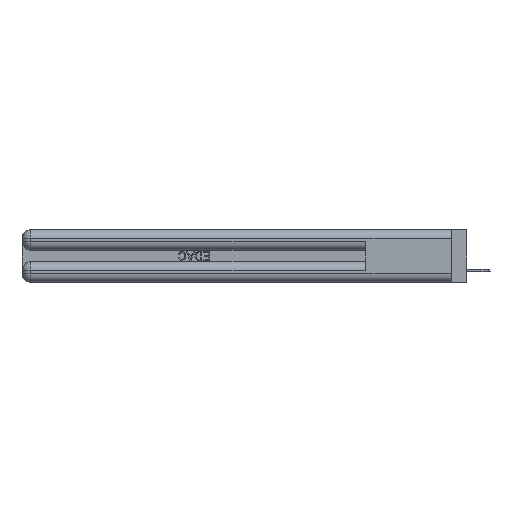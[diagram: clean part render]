
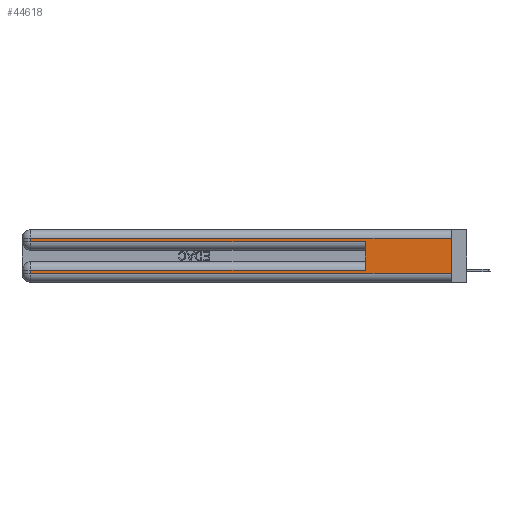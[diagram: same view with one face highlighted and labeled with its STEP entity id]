
A CAD part, left-side view. The second image highlights one B-rep face of the part: STEP entity #44618.
In plain terms, the highlighted planar face has unit normal (-1, 0, 0).
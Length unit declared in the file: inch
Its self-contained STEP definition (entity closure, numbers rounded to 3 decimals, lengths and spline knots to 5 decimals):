
#7 = EDGE_CURVE ( 'NONE', #6114, #13616, #32030, .T. ) ;
#2860 = DIRECTION ( 'NONE',  ( 0., 0., -1. ) ) ;
#5725 = VERTEX_POINT ( 'NONE', #36830 ) ;
#6114 = VERTEX_POINT ( 'NONE', #42309 ) ;
#8122 = EDGE_LOOP ( 'NONE', ( #51511, #28644, #48991, #49494, #27623, #25606, #29143, #9548 ) ) ;
#8180 = LINE ( 'NONE', #36721, #25839 ) ;
#8453 = VECTOR ( 'NONE', #35590, 39.37008 ) ;
#9548 = ORIENTED_EDGE ( 'NONE', *, *, #47513, .T. ) ;
#10100 = CARTESIAN_POINT ( 'NONE',  ( 0., 2.94, 0.37 ) ) ;
#11999 = EDGE_CURVE ( 'NONE', #47653, #46898, #13124, .T. ) ;
#12465 = VECTOR ( 'NONE', #18712, 39.37008 ) ;
#13124 = LINE ( 'NONE', #14796, #12465 ) ;
#13616 = VERTEX_POINT ( 'NONE', #33206 ) ;
#14796 = CARTESIAN_POINT ( 'NONE',  ( 0., 0., 0.285 ) ) ;
#15668 = VECTOR ( 'NONE', #39580, 39.37008 ) ;
#16251 = FACE_OUTER_BOUND ( 'NONE', #8122, .T. ) ;
#17069 = VECTOR ( 'NONE', #31730, 39.37008 ) ;
#17251 = CARTESIAN_POINT ( 'NONE',  ( 0., 2.94, 0.285 ) ) ;
#17405 = EDGE_CURVE ( 'NONE', #5725, #22506, #32614, .T. ) ;
#18120 = VERTEX_POINT ( 'NONE', #48174 ) ;
#18712 = DIRECTION ( 'NONE',  ( 0., -1., 0. ) ) ;
#22506 = VERTEX_POINT ( 'NONE', #42039 ) ;
#23694 = LINE ( 'NONE', #38310, #8453 ) ;
#24820 = EDGE_CURVE ( 'NONE', #13616, #44386, #34417, .T. ) ;
#24908 = EDGE_CURVE ( 'NONE', #6114, #46898, #23694, .T. ) ;
#25606 = ORIENTED_EDGE ( 'NONE', *, *, #7, .T. ) ;
#25839 = VECTOR ( 'NONE', #28259, 39.37008 ) ;
#27623 = ORIENTED_EDGE ( 'NONE', *, *, #24908, .F. ) ;
#27750 = CARTESIAN_POINT ( 'NONE',  ( 0., 2.94, 0.37 ) ) ;
#28259 = DIRECTION ( 'NONE',  ( 0., 0., -1. ) ) ;
#28539 = EDGE_CURVE ( 'NONE', #22506, #47653, #52403, .T. ) ;
#28644 = ORIENTED_EDGE ( 'NONE', *, *, #17405, .T. ) ;
#29143 = ORIENTED_EDGE ( 'NONE', *, *, #24820, .T. ) ;
#31730 = DIRECTION ( 'NONE',  ( 0., -1., 0. ) ) ;
#32030 = LINE ( 'NONE', #43398, #47993 ) ;
#32614 = LINE ( 'NONE', #51875, #15668 ) ;
#33206 = CARTESIAN_POINT ( 'NONE',  ( 0., 2.94, 0.085 ) ) ;
#33969 = DIRECTION ( 'NONE',  ( 1., 0., 0. ) ) ;
#34417 = LINE ( 'NONE', #27750, #50307 ) ;
#34623 = AXIS2_PLACEMENT_3D ( 'NONE', #49252, #33969, #50313 ) ;
#35590 = DIRECTION ( 'NONE',  ( 0., 0., 1. ) ) ;
#36721 = CARTESIAN_POINT ( 'NONE',  ( 0., 0., 0.37 ) ) ;
#36725 = LINE ( 'NONE', #44686, #17069 ) ;
#36830 = CARTESIAN_POINT ( 'NONE',  ( 0., 0., 0.31 ) ) ;
#38310 = CARTESIAN_POINT ( 'NONE',  ( 0., 0.6, 0.145 ) ) ;
#39560 = CARTESIAN_POINT ( 'NONE',  ( 0., 2.94, 0.06 ) ) ;
#39580 = DIRECTION ( 'NONE',  ( 0., 1., 0. ) ) ;
#39626 = DIRECTION ( 'NONE',  ( 0., 1., 0. ) ) ;
#42039 = CARTESIAN_POINT ( 'NONE',  ( 0., 2.94, 0.31 ) ) ;
#42309 = CARTESIAN_POINT ( 'NONE',  ( 0., 0.6, 0.085 ) ) ;
#43398 = CARTESIAN_POINT ( 'NONE',  ( 0., 0., 0.085 ) ) ;
#44386 = VERTEX_POINT ( 'NONE', #39560 ) ;
#44618 = ADVANCED_FACE ( 'NONE', ( #16251 ), #45506, .F. ) ;
#44686 = CARTESIAN_POINT ( 'NONE',  ( 0., 0., 0.06 ) ) ;
#45071 = CARTESIAN_POINT ( 'NONE',  ( 0., 0.6, 0.285 ) ) ;
#45347 = VECTOR ( 'NONE', #46776, 39.37008 ) ;
#45506 = PLANE ( 'NONE',  #34623 ) ;
#46776 = DIRECTION ( 'NONE',  ( 0., 0., -1. ) ) ;
#46898 = VERTEX_POINT ( 'NONE', #45071 ) ;
#47513 = EDGE_CURVE ( 'NONE', #44386, #18120, #36725, .T. ) ;
#47653 = VERTEX_POINT ( 'NONE', #17251 ) ;
#47993 = VECTOR ( 'NONE', #39626, 39.37008 ) ;
#48174 = CARTESIAN_POINT ( 'NONE',  ( 0., 0., 0.06 ) ) ;
#48792 = EDGE_CURVE ( 'NONE', #5725, #18120, #8180, .T. ) ;
#48991 = ORIENTED_EDGE ( 'NONE', *, *, #28539, .T. ) ;
#49252 = CARTESIAN_POINT ( 'NONE',  ( 0., 0., 0.37 ) ) ;
#49494 = ORIENTED_EDGE ( 'NONE', *, *, #11999, .T. ) ;
#50307 = VECTOR ( 'NONE', #2860, 39.37008 ) ;
#50313 = DIRECTION ( 'NONE',  ( 0., 0., -1. ) ) ;
#51511 = ORIENTED_EDGE ( 'NONE', *, *, #48792, .F. ) ;
#51875 = CARTESIAN_POINT ( 'NONE',  ( 0., 0., 0.31 ) ) ;
#52403 = LINE ( 'NONE', #10100, #45347 ) ;
